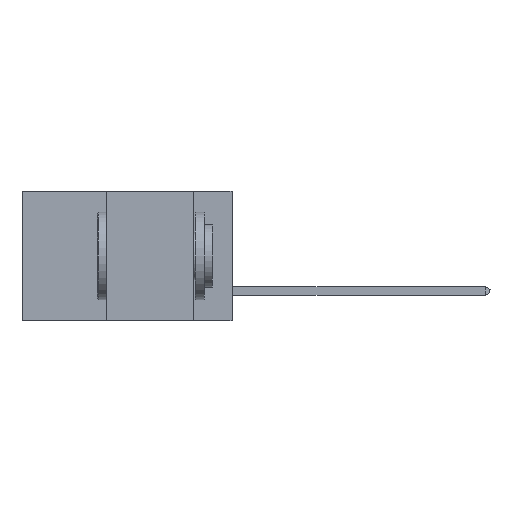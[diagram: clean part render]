
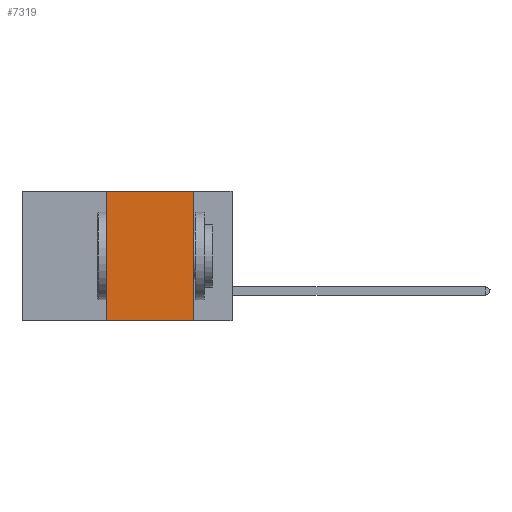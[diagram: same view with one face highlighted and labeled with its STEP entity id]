
A CAD part, left-side view. The second image highlights one B-rep face of the part: STEP entity #7319.
In plain terms, the highlighted planar face has unit normal (-1, 0, 0).
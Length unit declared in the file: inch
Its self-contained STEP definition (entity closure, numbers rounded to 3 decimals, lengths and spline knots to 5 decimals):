
#364 = ORIENTED_EDGE ( 'NONE', *, *, #11895, .F. ) ;
#665 = VERTEX_POINT ( 'NONE', #8209 ) ;
#672 = VECTOR ( 'NONE', #5089, 39.37008 ) ;
#909 = EDGE_LOOP ( 'NONE', ( #6685, #1079, #364, #11519 ) ) ;
#1011 = VERTEX_POINT ( 'NONE', #4483 ) ;
#1079 = ORIENTED_EDGE ( 'NONE', *, *, #11552, .F. ) ;
#1653 = CARTESIAN_POINT ( 'NONE',  ( 0., 0.6, 0. ) ) ;
#2900 = DIRECTION ( 'NONE',  ( 0., -1., 0. ) ) ;
#3950 = VERTEX_POINT ( 'NONE', #6367 ) ;
#4160 = VECTOR ( 'NONE', #2900, 39.37008 ) ;
#4472 = DIRECTION ( 'NONE',  ( 0., -1., 0. ) ) ;
#4483 = CARTESIAN_POINT ( 'NONE',  ( 0., 0.11, 0. ) ) ;
#4963 = CARTESIAN_POINT ( 'NONE',  ( 0., 0.6, 0. ) ) ;
#4984 = DIRECTION ( 'NONE',  ( 0., 0., 1. ) ) ;
#5089 = DIRECTION ( 'NONE',  ( 0., 0., -1. ) ) ;
#5850 = PLANE ( 'NONE',  #9033 ) ;
#5888 = DIRECTION ( 'NONE',  ( 0., 0., -1. ) ) ;
#6367 = CARTESIAN_POINT ( 'NONE',  ( 0., 0.11, -0.37 ) ) ;
#6510 = LINE ( 'NONE', #1653, #4160 ) ;
#6627 = LINE ( 'NONE', #9891, #672 ) ;
#6685 = ORIENTED_EDGE ( 'NONE', *, *, #7049, .F. ) ;
#7049 = EDGE_CURVE ( 'NONE', #1011, #3950, #6627, .T. ) ;
#7224 = CARTESIAN_POINT ( 'NONE',  ( 0., 0.6, -0.37 ) ) ;
#7287 = CARTESIAN_POINT ( 'NONE',  ( 0., 0.36, -0.37 ) ) ;
#7319 = ADVANCED_FACE ( 'NONE', ( #9662 ), #5850, .F. ) ;
#8209 = CARTESIAN_POINT ( 'NONE',  ( 0., 0.36, 0. ) ) ;
#8374 = VECTOR ( 'NONE', #4984, 39.37008 ) ;
#9011 = EDGE_CURVE ( 'NONE', #11218, #3950, #9082, .T. ) ;
#9033 = AXIS2_PLACEMENT_3D ( 'NONE', #4963, #11520, #5888 ) ;
#9070 = VECTOR ( 'NONE', #4472, 39.37008 ) ;
#9082 = LINE ( 'NONE', #7224, #9070 ) ;
#9662 = FACE_OUTER_BOUND ( 'NONE', #909, .T. ) ;
#9712 = CARTESIAN_POINT ( 'NONE',  ( 0., 0.36, 0. ) ) ;
#9891 = CARTESIAN_POINT ( 'NONE',  ( 0., 0.11, 0. ) ) ;
#11218 = VERTEX_POINT ( 'NONE', #7287 ) ;
#11414 = LINE ( 'NONE', #9712, #8374 ) ;
#11519 = ORIENTED_EDGE ( 'NONE', *, *, #9011, .T. ) ;
#11520 = DIRECTION ( 'NONE',  ( 1., 0., 0. ) ) ;
#11552 = EDGE_CURVE ( 'NONE', #665, #1011, #6510, .T. ) ;
#11895 = EDGE_CURVE ( 'NONE', #11218, #665, #11414, .T. ) ;
